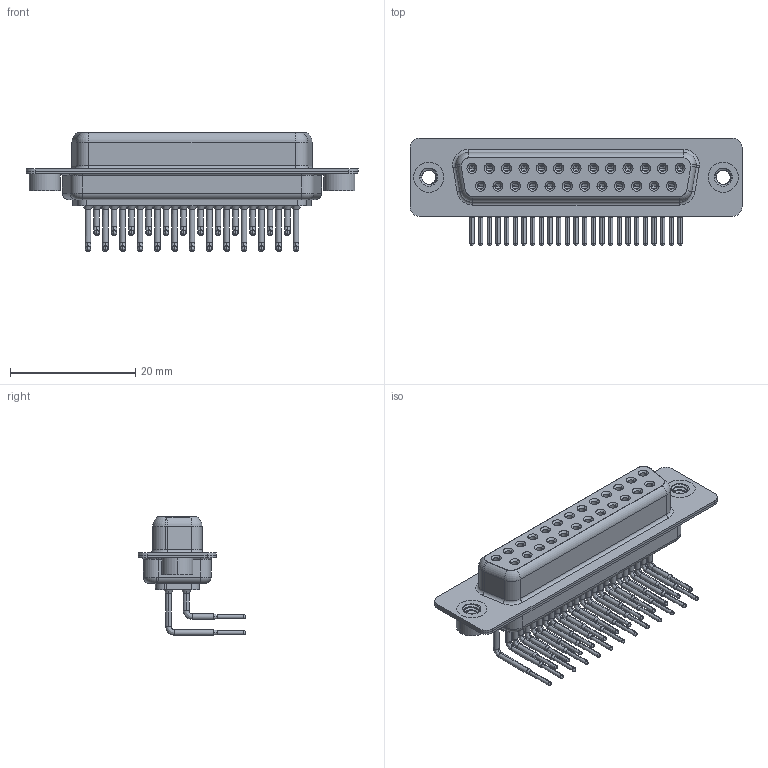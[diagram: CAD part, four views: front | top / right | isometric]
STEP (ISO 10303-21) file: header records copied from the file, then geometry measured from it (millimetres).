
FILE_DESCRIPTION (( 'STEP AP203' ), '1' );
FILE_NAME ('630-M25-640-WT2.STEP', '2018-09-26T02:53:45', ( '' ), ( '' ), 'SwSTEP 2.0', 'SolidWorks 2016', '' );
FILE_SCHEMA (( 'CONFIG_CONTROL_DESIGN' ));
Length unit declared in the file: millimetre
Products named in the file (7): 630M Shell Rear_25 Contacts; 630M Contact Row 1; 630M Contact Row 2; 630M 4-40 Threaded Rivet; 630-M25-640-WT2; 630M Housing_25 Contacts; 630M Shell Front_25 Contacts
Assembly tree (30 placements, depth 2):
  630-M25-640-WT2
    630M Housing_25 Contacts
    630M Shell Front_25 Contacts
    630M Shell Rear_25 Contacts
    630M Contact Row 1  x13
    630M Contact Row 2  x12
    630M 4-40 Threaded Rivet  x2
Bounding box: 53.05 x 17.2 x 18.99 mm (x, y, z)
Volume: 3898.1 mm3; surface area: 9728.5 mm2
Topology: 30 solids, 30 shells, 1604 faces, 4062 edges, 2554 vertices
Faces by surface type: cylinder 712, plane 442, cone 281, bspline 106, torus 63
Entity records: 21982 total; most frequent: CARTESIAN_POINT 5009, DIRECTION 3599, ORIENTED_EDGE 3022, EDGE_CURVE 1511, AXIS2_PLACEMENT_3D 1510, VERTEX_POINT 960, CIRCLE 837, EDGE_LOOP 803
